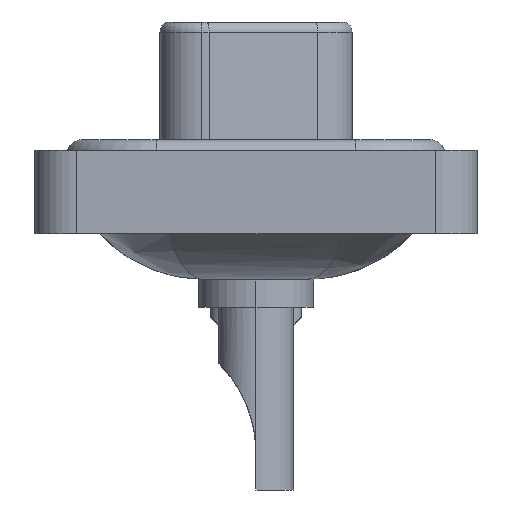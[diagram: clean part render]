
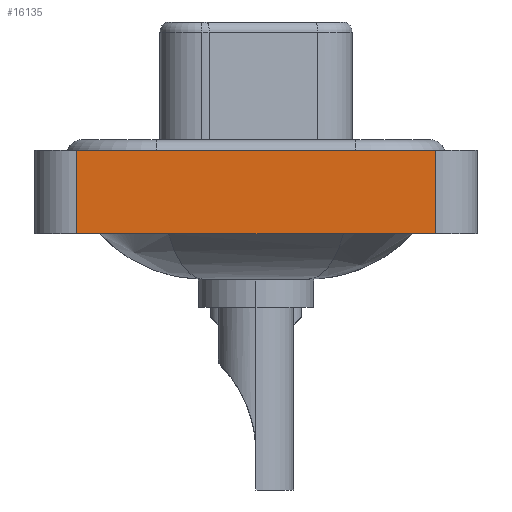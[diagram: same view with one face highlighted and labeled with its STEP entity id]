
A CAD part, left-side view. The second image highlights one B-rep face of the part: STEP entity #16135.
In plain terms, the highlighted planar face has unit normal (-1, 0, 0).
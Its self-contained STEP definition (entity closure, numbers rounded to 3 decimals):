
#1198 = CARTESIAN_POINT ( 'NONE',  ( -7.3, -8.55, -3.6 ) ) ;
#1289 = DIRECTION ( 'NONE',  ( 0., 0., 1. ) ) ;
#1381 = CARTESIAN_POINT ( 'NONE',  ( -7.3, -8.55, 0.4 ) ) ;
#1414 = DIRECTION ( 'NONE',  ( 0., 0., 1. ) ) ;
#1842 = CARTESIAN_POINT ( 'NONE',  ( -7.3, -8.55, 0.4 ) ) ;
#2363 = ORIENTED_EDGE ( 'NONE', *, *, #7304, .T. ) ;
#3898 = CARTESIAN_POINT ( 'NONE',  ( -7.3, 8.55, 0.4 ) ) ;
#4314 = VECTOR ( 'NONE', #7954, 1000. ) ;
#4420 = FACE_OUTER_BOUND ( 'NONE', #6679, .T. ) ;
#5434 = DIRECTION ( 'NONE',  ( 0., -1., 0. ) ) ;
#5599 = VECTOR ( 'NONE', #12714, 1000. ) ;
#6173 = VERTEX_POINT ( 'NONE', #7044 ) ;
#6257 = LINE ( 'NONE', #1842, #4314 ) ;
#6558 = EDGE_CURVE ( 'NONE', #6173, #9791, #14700, .T. ) ;
#6679 = EDGE_LOOP ( 'NONE', ( #14383, #9317, #17709, #2363 ) ) ;
#7044 = CARTESIAN_POINT ( 'NONE',  ( -7.3, -8.55, -3.6 ) ) ;
#7131 = VERTEX_POINT ( 'NONE', #3898 ) ;
#7304 = EDGE_CURVE ( 'NONE', #7963, #6173, #16033, .T. ) ;
#7954 = DIRECTION ( 'NONE',  ( 0., -1., 0. ) ) ;
#7963 = VERTEX_POINT ( 'NONE', #13688 ) ;
#9237 = CARTESIAN_POINT ( 'NONE',  ( -7.3, -8.55, -3.6 ) ) ;
#9317 = ORIENTED_EDGE ( 'NONE', *, *, #11993, .F. ) ;
#9791 = VERTEX_POINT ( 'NONE', #1381 ) ;
#11546 = VECTOR ( 'NONE', #1289, 1000. ) ;
#11993 = EDGE_CURVE ( 'NONE', #7131, #9791, #6257, .T. ) ;
#12615 = EDGE_CURVE ( 'NONE', #7963, #7131, #15427, .T. ) ;
#12714 = DIRECTION ( 'NONE',  ( 0., 0., 1. ) ) ;
#12801 = CARTESIAN_POINT ( 'NONE',  ( -7.3, -8.55, -3.6 ) ) ;
#13688 = CARTESIAN_POINT ( 'NONE',  ( -7.3, 8.55, -3.6 ) ) ;
#14383 = ORIENTED_EDGE ( 'NONE', *, *, #6558, .T. ) ;
#14700 = LINE ( 'NONE', #1198, #11546 ) ;
#15082 = VECTOR ( 'NONE', #5434, 1000. ) ;
#15394 = DIRECTION ( 'NONE',  ( -1., 0., 0. ) ) ;
#15427 = LINE ( 'NONE', #17648, #5599 ) ;
#16033 = LINE ( 'NONE', #12801, #15082 ) ;
#16135 = ADVANCED_FACE ( 'NONE', ( #4420 ), #16921, .T. ) ;
#16921 = PLANE ( 'NONE',  #18760 ) ;
#17648 = CARTESIAN_POINT ( 'NONE',  ( -7.3, 8.55, -3.6 ) ) ;
#17709 = ORIENTED_EDGE ( 'NONE', *, *, #12615, .F. ) ;
#18760 = AXIS2_PLACEMENT_3D ( 'NONE', #9237, #15394, #1414 ) ;
